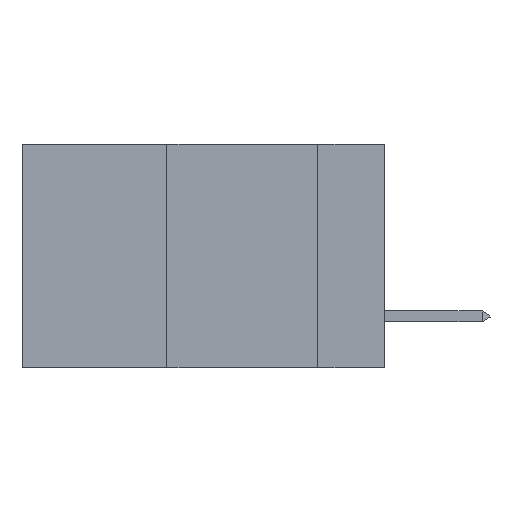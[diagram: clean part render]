
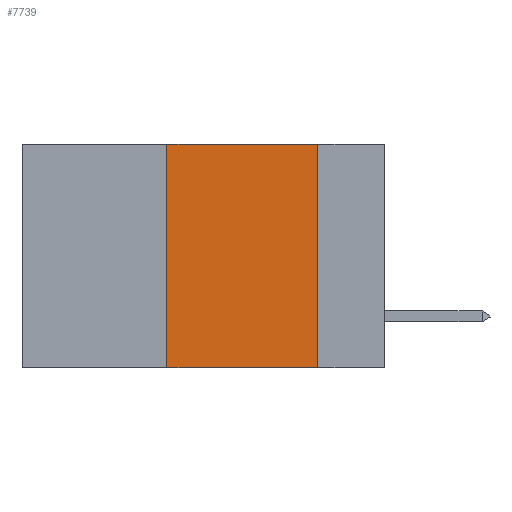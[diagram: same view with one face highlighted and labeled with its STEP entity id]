
A CAD part, left-side view. The second image highlights one B-rep face of the part: STEP entity #7739.
In plain terms, the highlighted planar face has unit normal (-1, 0, 0).
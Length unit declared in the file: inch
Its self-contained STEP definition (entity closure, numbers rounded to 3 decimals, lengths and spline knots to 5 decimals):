
#234 = DIRECTION ( 'NONE',  ( 0., 0., -1. ) ) ;
#1618 = EDGE_CURVE ( 'NONE', #7051, #2095, #13782, .T. ) ;
#2095 = VERTEX_POINT ( 'NONE', #3816 ) ;
#2946 = CARTESIAN_POINT ( 'NONE',  ( 0., 0.6, 0. ) ) ;
#3006 = CARTESIAN_POINT ( 'NONE',  ( 0., 0.36, 0. ) ) ;
#3483 = EDGE_CURVE ( 'NONE', #8615, #2095, #12872, .T. ) ;
#3805 = VECTOR ( 'NONE', #234, 39.37008 ) ;
#3807 = AXIS2_PLACEMENT_3D ( 'NONE', #8537, #8663, #15241 ) ;
#3816 = CARTESIAN_POINT ( 'NONE',  ( 0., 0.11, -0.37 ) ) ;
#5887 = EDGE_CURVE ( 'NONE', #8615, #11013, #13436, .T. ) ;
#5957 = EDGE_CURVE ( 'NONE', #11013, #7051, #7021, .T. ) ;
#7021 = LINE ( 'NONE', #2946, #9783 ) ;
#7051 = VERTEX_POINT ( 'NONE', #12497 ) ;
#7071 = DIRECTION ( 'NONE',  ( 0., -1., 0. ) ) ;
#7306 = PLANE ( 'NONE',  #3807 ) ;
#7508 = DIRECTION ( 'NONE',  ( 0., -1., 0. ) ) ;
#7739 = ADVANCED_FACE ( 'NONE', ( #17189 ), #7306, .F. ) ;
#8282 = CARTESIAN_POINT ( 'NONE',  ( 0., 0.11, 0. ) ) ;
#8537 = CARTESIAN_POINT ( 'NONE',  ( 0., 0.6, 0. ) ) ;
#8615 = VERTEX_POINT ( 'NONE', #16260 ) ;
#8649 = ORIENTED_EDGE ( 'NONE', *, *, #1618, .F. ) ;
#8663 = DIRECTION ( 'NONE',  ( 1., 0., 0. ) ) ;
#9783 = VECTOR ( 'NONE', #7071, 39.37008 ) ;
#11013 = VERTEX_POINT ( 'NONE', #16499 ) ;
#12239 = ORIENTED_EDGE ( 'NONE', *, *, #5957, .F. ) ;
#12348 = EDGE_LOOP ( 'NONE', ( #8649, #12239, #16017, #14268 ) ) ;
#12497 = CARTESIAN_POINT ( 'NONE',  ( 0., 0.11, 0. ) ) ;
#12872 = LINE ( 'NONE', #16861, #15646 ) ;
#13436 = LINE ( 'NONE', #3006, #16413 ) ;
#13782 = LINE ( 'NONE', #8282, #3805 ) ;
#14268 = ORIENTED_EDGE ( 'NONE', *, *, #3483, .T. ) ;
#15171 = DIRECTION ( 'NONE',  ( 0., 0., 1. ) ) ;
#15241 = DIRECTION ( 'NONE',  ( 0., 0., -1. ) ) ;
#15646 = VECTOR ( 'NONE', #7508, 39.37008 ) ;
#16017 = ORIENTED_EDGE ( 'NONE', *, *, #5887, .F. ) ;
#16260 = CARTESIAN_POINT ( 'NONE',  ( 0., 0.36, -0.37 ) ) ;
#16413 = VECTOR ( 'NONE', #15171, 39.37008 ) ;
#16499 = CARTESIAN_POINT ( 'NONE',  ( 0., 0.36, 0. ) ) ;
#16861 = CARTESIAN_POINT ( 'NONE',  ( 0., 0.6, -0.37 ) ) ;
#17189 = FACE_OUTER_BOUND ( 'NONE', #12348, .T. ) ;
